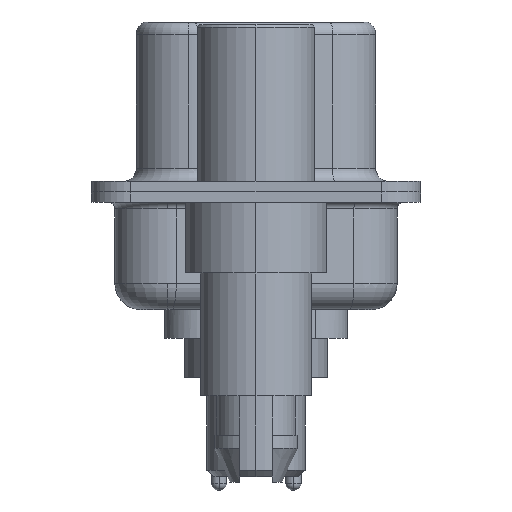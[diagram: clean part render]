
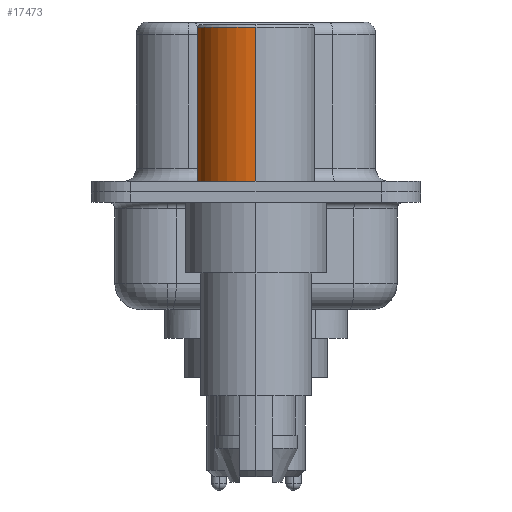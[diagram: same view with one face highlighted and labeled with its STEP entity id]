
A CAD part, left-side view. The second image highlights one B-rep face of the part: STEP entity #17473.
In plain terms, the highlighted cylindrical face has radius 2.25 mm (diameter 4.5 mm), a partial arc.
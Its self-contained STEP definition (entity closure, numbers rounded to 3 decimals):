
#491 = CARTESIAN_POINT ( 'NONE',  ( 0., 0., 0.4 ) ) ;
#2180 = DIRECTION ( 'NONE',  ( 1., 0., 0. ) ) ;
#2996 = DIRECTION ( 'NONE',  ( 0., 0., 1. ) ) ;
#3419 = VECTOR ( 'NONE', #2996, 1000. ) ;
#4841 = CARTESIAN_POINT ( 'NONE',  ( 0., 0., 0.581 ) ) ;
#5689 = CARTESIAN_POINT ( 'NONE',  ( 0., 0., 6.3 ) ) ;
#6535 = ORIENTED_EDGE ( 'NONE', *, *, #11903, .T. ) ;
#7297 = DIRECTION ( 'NONE',  ( 1., 0., 0. ) ) ;
#7378 = EDGE_LOOP ( 'NONE', ( #6535, #9197, #8723, #14981 ) ) ;
#8574 = FACE_OUTER_BOUND ( 'NONE', #7378, .T. ) ;
#8723 = ORIENTED_EDGE ( 'NONE', *, *, #14581, .F. ) ;
#9033 = CARTESIAN_POINT ( 'NONE',  ( -2.25, 0., 0.581 ) ) ;
#9166 = AXIS2_PLACEMENT_3D ( 'NONE', #491, #11785, #2180 ) ;
#9197 = ORIENTED_EDGE ( 'NONE', *, *, #20710, .T. ) ;
#10615 = AXIS2_PLACEMENT_3D ( 'NONE', #4841, #17461, #11219 ) ;
#10932 = LINE ( 'NONE', #12610, #3419 ) ;
#11007 = VERTEX_POINT ( 'NONE', #18665 ) ;
#11219 = DIRECTION ( 'NONE',  ( 1., 0., 0. ) ) ;
#11399 = CIRCLE ( 'NONE', #13244, 2.25 ) ;
#11536 = CARTESIAN_POINT ( 'NONE',  ( -2.25, 0., 0.4 ) ) ;
#11655 = LINE ( 'NONE', #9033, #19503 ) ;
#11785 = DIRECTION ( 'NONE',  ( 0., 0., 1. ) ) ;
#11872 = CIRCLE ( 'NONE', #9166, 2.25 ) ;
#11903 = EDGE_CURVE ( 'NONE', #11007, #16985, #11872, .T. ) ;
#12610 = CARTESIAN_POINT ( 'NONE',  ( 2.25, 0., 0.581 ) ) ;
#12743 = VERTEX_POINT ( 'NONE', #17706 ) ;
#13244 = AXIS2_PLACEMENT_3D ( 'NONE', #5689, #16664, #7297 ) ;
#14581 = EDGE_CURVE ( 'NONE', #19688, #12743, #11399, .T. ) ;
#14981 = ORIENTED_EDGE ( 'NONE', *, *, #20455, .F. ) ;
#16425 = CYLINDRICAL_SURFACE ( 'NONE', #10615, 2.25 ) ;
#16664 = DIRECTION ( 'NONE',  ( 0., 0., 1. ) ) ;
#16985 = VERTEX_POINT ( 'NONE', #11536 ) ;
#17461 = DIRECTION ( 'NONE',  ( 0., 0., 1. ) ) ;
#17473 = ADVANCED_FACE ( 'NONE', ( #8574 ), #16425, .T. ) ;
#17529 = CARTESIAN_POINT ( 'NONE',  ( 2.25, 0., 6.3 ) ) ;
#17706 = CARTESIAN_POINT ( 'NONE',  ( -2.25, 0., 6.3 ) ) ;
#18424 = DIRECTION ( 'NONE',  ( 0., 0., 1. ) ) ;
#18665 = CARTESIAN_POINT ( 'NONE',  ( 2.25, 0., 0.4 ) ) ;
#19503 = VECTOR ( 'NONE', #18424, 1000. ) ;
#19688 = VERTEX_POINT ( 'NONE', #17529 ) ;
#20455 = EDGE_CURVE ( 'NONE', #11007, #19688, #10932, .T. ) ;
#20710 = EDGE_CURVE ( 'NONE', #16985, #12743, #11655, .T. ) ;
